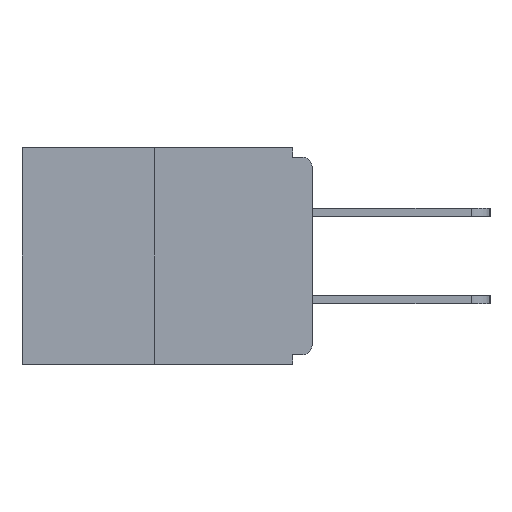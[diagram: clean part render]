
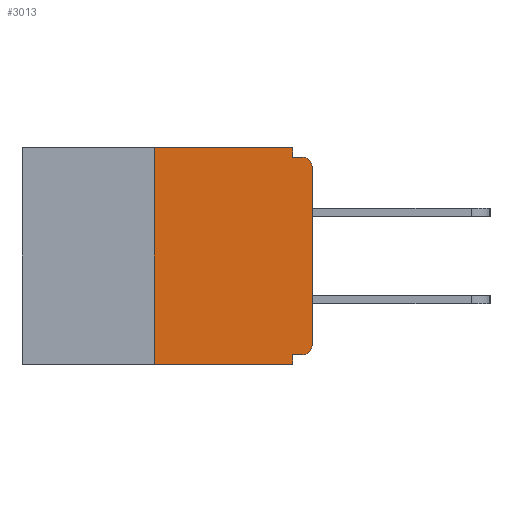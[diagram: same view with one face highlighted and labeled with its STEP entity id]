
A CAD part, left-side view. The second image highlights one B-rep face of the part: STEP entity #3013.
In plain terms, the highlighted planar face has unit normal (-1, 0, 0).
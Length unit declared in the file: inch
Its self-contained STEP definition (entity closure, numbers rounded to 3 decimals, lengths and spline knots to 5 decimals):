
#174 = CARTESIAN_POINT ( 'NONE',  ( 0., 0., -0.03 ) ) ;
#605 = DIRECTION ( 'NONE',  ( -1., 0., 0. ) ) ;
#698 = CIRCLE ( 'NONE', #14876, 0.015 ) ;
#1363 = LINE ( 'NONE', #1479, #8799 ) ;
#1479 = CARTESIAN_POINT ( 'NONE',  ( 0., 0.25, 0. ) ) ;
#1882 = CARTESIAN_POINT ( 'NONE',  ( 0., 0., -0.015 ) ) ;
#2588 = ORIENTED_EDGE ( 'NONE', *, *, #20566, .F. ) ;
#2653 = VERTEX_POINT ( 'NONE', #7829 ) ;
#2973 = PLANE ( 'NONE',  #16959 ) ;
#3013 = ADVANCED_FACE ( 'NONE', ( #12492 ), #2973, .F. ) ;
#3186 = CARTESIAN_POINT ( 'NONE',  ( 0., 0.46, -0.343 ) ) ;
#3565 = CARTESIAN_POINT ( 'NONE',  ( 0., 0.015, -0.03 ) ) ;
#3828 = CIRCLE ( 'NONE', #5162, 0.015 ) ;
#3974 = CARTESIAN_POINT ( 'NONE',  ( 0., 0.015, -0.313 ) ) ;
#4147 = VERTEX_POINT ( 'NONE', #17770 ) ;
#4162 = ORIENTED_EDGE ( 'NONE', *, *, #17302, .F. ) ;
#4304 = LINE ( 'NONE', #20526, #8573 ) ;
#4399 = EDGE_CURVE ( 'NONE', #2653, #6445, #3828, .T. ) ;
#4406 = DIRECTION ( 'NONE',  ( 0., 0., 1. ) ) ;
#4596 = VERTEX_POINT ( 'NONE', #174 ) ;
#4776 = VECTOR ( 'NONE', #9626, 39.37008 ) ;
#5162 = AXIS2_PLACEMENT_3D ( 'NONE', #3974, #605, #8818 ) ;
#5314 = DIRECTION ( 'NONE',  ( -1., 0., 0. ) ) ;
#5590 = CARTESIAN_POINT ( 'NONE',  ( 0., 0.25, 0. ) ) ;
#5716 = VERTEX_POINT ( 'NONE', #19218 ) ;
#6215 = CARTESIAN_POINT ( 'NONE',  ( 0., 0., -0.313 ) ) ;
#6445 = VERTEX_POINT ( 'NONE', #6215 ) ;
#6674 = VERTEX_POINT ( 'NONE', #11909 ) ;
#6684 = CARTESIAN_POINT ( 'NONE',  ( 0., 0., -0.328 ) ) ;
#6694 = ORIENTED_EDGE ( 'NONE', *, *, #12194, .T. ) ;
#7335 = DIRECTION ( 'NONE',  ( 0., 0., -1. ) ) ;
#7829 = CARTESIAN_POINT ( 'NONE',  ( 0., 0.015, -0.328 ) ) ;
#7965 = ORIENTED_EDGE ( 'NONE', *, *, #16154, .T. ) ;
#8276 = ORIENTED_EDGE ( 'NONE', *, *, #13344, .T. ) ;
#8479 = EDGE_CURVE ( 'NONE', #5716, #4147, #12878, .T. ) ;
#8573 = VECTOR ( 'NONE', #7335, 39.37008 ) ;
#8575 = EDGE_CURVE ( 'NONE', #11108, #15072, #18173, .T. ) ;
#8613 = DIRECTION ( 'NONE',  ( 0., -1., 0. ) ) ;
#8622 = LINE ( 'NONE', #3186, #4776 ) ;
#8799 = VECTOR ( 'NONE', #9607, 39.37008 ) ;
#8818 = DIRECTION ( 'NONE',  ( 0., 0., -1. ) ) ;
#9209 = DIRECTION ( 'NONE',  ( 0., 0., -1. ) ) ;
#9607 = DIRECTION ( 'NONE',  ( 0., 0., 1. ) ) ;
#9626 = DIRECTION ( 'NONE',  ( 0., -1., 0. ) ) ;
#9876 = ORIENTED_EDGE ( 'NONE', *, *, #19610, .F. ) ;
#10527 = VECTOR ( 'NONE', #11215, 39.37008 ) ;
#10856 = DIRECTION ( 'NONE',  ( 0., 0., -1. ) ) ;
#10979 = CARTESIAN_POINT ( 'NONE',  ( 0., 0.031, -0.343 ) ) ;
#11108 = VERTEX_POINT ( 'NONE', #16909 ) ;
#11215 = DIRECTION ( 'NONE',  ( 0., -1., 0. ) ) ;
#11909 = CARTESIAN_POINT ( 'NONE',  ( 0., 0.031, 0. ) ) ;
#12129 = ORIENTED_EDGE ( 'NONE', *, *, #4399, .T. ) ;
#12194 = EDGE_CURVE ( 'NONE', #4596, #15072, #698, .T. ) ;
#12283 = CARTESIAN_POINT ( 'NONE',  ( 0., 0.25, -0.343 ) ) ;
#12399 = DIRECTION ( 'NONE',  ( 1., 0., 0. ) ) ;
#12492 = FACE_OUTER_BOUND ( 'NONE', #15429, .T. ) ;
#12878 = LINE ( 'NONE', #10979, #15322 ) ;
#12938 = VECTOR ( 'NONE', #8613, 39.37008 ) ;
#13003 = VERTEX_POINT ( 'NONE', #12283 ) ;
#13344 = EDGE_CURVE ( 'NONE', #13003, #4147, #8622, .T. ) ;
#14081 = ORIENTED_EDGE ( 'NONE', *, *, #17396, .F. ) ;
#14363 = VECTOR ( 'NONE', #4406, 39.37008 ) ;
#14501 = CARTESIAN_POINT ( 'NONE',  ( 0., 0.46, 0. ) ) ;
#14876 = AXIS2_PLACEMENT_3D ( 'NONE', #3565, #5314, #15087 ) ;
#15072 = VERTEX_POINT ( 'NONE', #16856 ) ;
#15087 = DIRECTION ( 'NONE',  ( 0., 0., -1. ) ) ;
#15322 = VECTOR ( 'NONE', #10856, 39.37008 ) ;
#15429 = EDGE_LOOP ( 'NONE', ( #2588, #9876, #8276, #20638, #14081, #12129, #7965, #6694, #20475, #4162 ) ) ;
#15804 = CARTESIAN_POINT ( 'NONE',  ( 0., 0.46, 0. ) ) ;
#16102 = VECTOR ( 'NONE', #16161, 39.37008 ) ;
#16154 = EDGE_CURVE ( 'NONE', #6445, #4596, #18923, .T. ) ;
#16161 = DIRECTION ( 'NONE',  ( 0., 1., 0. ) ) ;
#16856 = CARTESIAN_POINT ( 'NONE',  ( 0., 0.015, -0.015 ) ) ;
#16909 = CARTESIAN_POINT ( 'NONE',  ( 0., 0.031, -0.015 ) ) ;
#16959 = AXIS2_PLACEMENT_3D ( 'NONE', #15804, #12399, #9209 ) ;
#17302 = EDGE_CURVE ( 'NONE', #6674, #11108, #4304, .T. ) ;
#17396 = EDGE_CURVE ( 'NONE', #2653, #5716, #19327, .T. ) ;
#17770 = CARTESIAN_POINT ( 'NONE',  ( 0., 0.031, -0.343 ) ) ;
#17806 = LINE ( 'NONE', #14501, #10527 ) ;
#17958 = VERTEX_POINT ( 'NONE', #5590 ) ;
#18173 = LINE ( 'NONE', #1882, #12938 ) ;
#18923 = LINE ( 'NONE', #20432, #14363 ) ;
#19218 = CARTESIAN_POINT ( 'NONE',  ( 0., 0.031, -0.328 ) ) ;
#19327 = LINE ( 'NONE', #6684, #16102 ) ;
#19610 = EDGE_CURVE ( 'NONE', #13003, #17958, #1363, .T. ) ;
#20432 = CARTESIAN_POINT ( 'NONE',  ( 0., 0., 0. ) ) ;
#20475 = ORIENTED_EDGE ( 'NONE', *, *, #8575, .F. ) ;
#20526 = CARTESIAN_POINT ( 'NONE',  ( 0., 0.031, 0. ) ) ;
#20566 = EDGE_CURVE ( 'NONE', #17958, #6674, #17806, .T. ) ;
#20638 = ORIENTED_EDGE ( 'NONE', *, *, #8479, .F. ) ;
